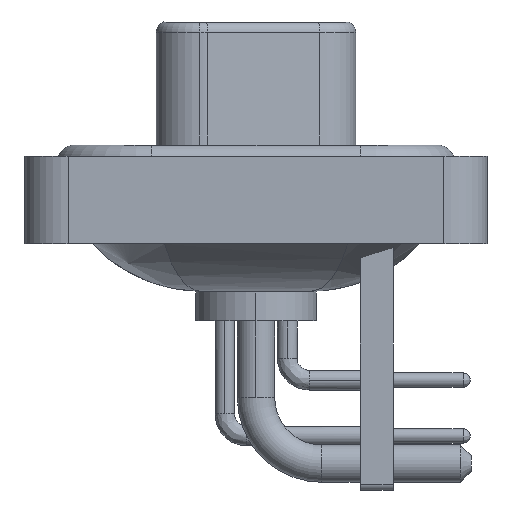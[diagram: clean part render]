
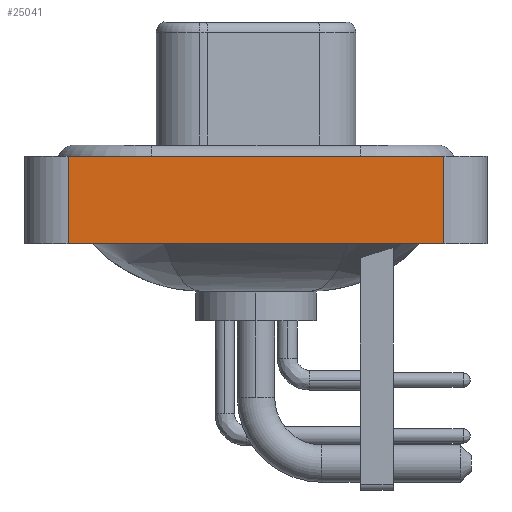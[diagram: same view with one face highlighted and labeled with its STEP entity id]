
A CAD part, left-side view. The second image highlights one B-rep face of the part: STEP entity #25041.
In plain terms, the highlighted planar face has unit normal (-1, 0, 0).
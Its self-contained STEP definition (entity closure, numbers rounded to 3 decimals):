
#782 = ORIENTED_EDGE ( 'NONE', *, *, #12304, .F. ) ;
#1064 = ORIENTED_EDGE ( 'NONE', *, *, #24957, .F. ) ;
#1564 = ORIENTED_EDGE ( 'NONE', *, *, #14218, .T. ) ;
#2368 = VERTEX_POINT ( 'NONE', #11714 ) ;
#2830 = DIRECTION ( 'NONE',  ( 0., -1., 0. ) ) ;
#3395 = DIRECTION ( 'NONE',  ( 0., 0., 1. ) ) ;
#3629 = VERTEX_POINT ( 'NONE', #23490 ) ;
#4366 = FACE_OUTER_BOUND ( 'NONE', #21346, .T. ) ;
#4507 = EDGE_CURVE ( 'NONE', #3629, #18058, #24359, .T. ) ;
#4776 = CARTESIAN_POINT ( 'NONE',  ( -7.3, -8.55, -3.6 ) ) ;
#4931 = VECTOR ( 'NONE', #9516, 1000. ) ;
#5416 = CARTESIAN_POINT ( 'NONE',  ( -7.3, 8.55, -3.6 ) ) ;
#5439 = VECTOR ( 'NONE', #3395, 1000. ) ;
#5723 = DIRECTION ( 'NONE',  ( 0., -1., 0. ) ) ;
#6791 = VECTOR ( 'NONE', #2830, 1000. ) ;
#6805 = CARTESIAN_POINT ( 'NONE',  ( -7.3, -8.55, -3.6 ) ) ;
#8217 = CARTESIAN_POINT ( 'NONE',  ( -7.3, -8.55, -3.6 ) ) ;
#9265 = LINE ( 'NONE', #5416, #4931 ) ;
#9516 = DIRECTION ( 'NONE',  ( 0., 0., 1. ) ) ;
#11714 = CARTESIAN_POINT ( 'NONE',  ( -7.3, 8.55, 0.4 ) ) ;
#12184 = DIRECTION ( 'NONE',  ( 0., 0., 1. ) ) ;
#12304 = EDGE_CURVE ( 'NONE', #2368, #21195, #21222, .T. ) ;
#14218 = EDGE_CURVE ( 'NONE', #18058, #21195, #18740, .T. ) ;
#17812 = DIRECTION ( 'NONE',  ( -1., 0., 0. ) ) ;
#18058 = VERTEX_POINT ( 'NONE', #22050 ) ;
#18674 = CARTESIAN_POINT ( 'NONE',  ( -7.3, -8.55, 0.4 ) ) ;
#18740 = LINE ( 'NONE', #4776, #5439 ) ;
#19652 = AXIS2_PLACEMENT_3D ( 'NONE', #8217, #17812, #12184 ) ;
#19984 = PLANE ( 'NONE',  #19652 ) ;
#20298 = VECTOR ( 'NONE', #5723, 1000. ) ;
#21175 = ORIENTED_EDGE ( 'NONE', *, *, #4507, .T. ) ;
#21195 = VERTEX_POINT ( 'NONE', #18674 ) ;
#21222 = LINE ( 'NONE', #21470, #20298 ) ;
#21346 = EDGE_LOOP ( 'NONE', ( #1564, #782, #1064, #21175 ) ) ;
#21470 = CARTESIAN_POINT ( 'NONE',  ( -7.3, -8.55, 0.4 ) ) ;
#22050 = CARTESIAN_POINT ( 'NONE',  ( -7.3, -8.55, -3.6 ) ) ;
#23490 = CARTESIAN_POINT ( 'NONE',  ( -7.3, 8.55, -3.6 ) ) ;
#24359 = LINE ( 'NONE', #6805, #6791 ) ;
#24957 = EDGE_CURVE ( 'NONE', #3629, #2368, #9265, .T. ) ;
#25041 = ADVANCED_FACE ( 'NONE', ( #4366 ), #19984, .T. ) ;
